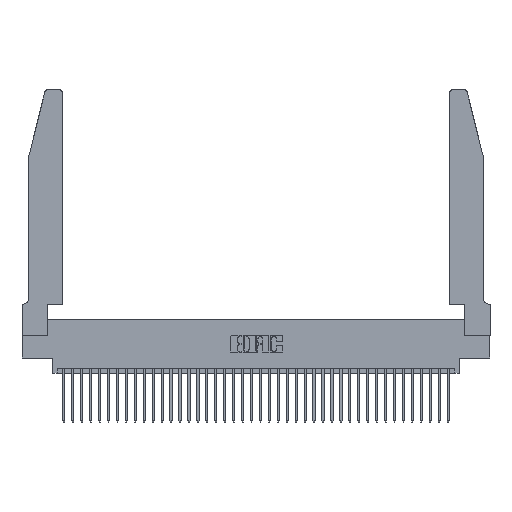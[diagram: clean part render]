
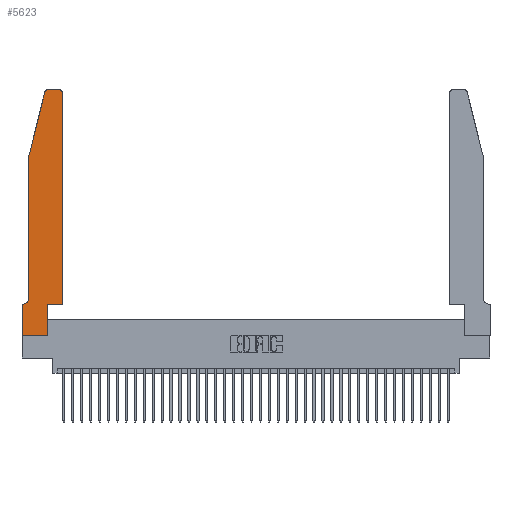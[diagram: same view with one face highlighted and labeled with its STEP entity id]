
A CAD part, top view. The second image highlights one B-rep face of the part: STEP entity #5623.
In plain terms, the highlighted planar face has unit normal (0, 0, 1).
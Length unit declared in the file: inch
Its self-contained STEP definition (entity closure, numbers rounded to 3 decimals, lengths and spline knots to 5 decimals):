
#653 = VERTEX_POINT ( 'NONE', #10343 ) ;
#885 = EDGE_CURVE ( 'NONE', #4570, #23562, #22742, .T. ) ;
#915 = ORIENTED_EDGE ( 'NONE', *, *, #18778, .T. ) ;
#2082 = VERTEX_POINT ( 'NONE', #32056 ) ;
#2391 = ORIENTED_EDGE ( 'NONE', *, *, #9731, .T. ) ;
#2848 = LINE ( 'NONE', #17155, #34085 ) ;
#3186 = AXIS2_PLACEMENT_3D ( 'NONE', #27260, #9106, #30260 ) ;
#3385 = EDGE_CURVE ( 'NONE', #26165, #33886, #33449, .T. ) ;
#4570 = VERTEX_POINT ( 'NONE', #22131 ) ;
#4640 = CARTESIAN_POINT ( 'NONE',  ( 0.4505, 0.35, 0.37 ) ) ;
#5017 = ORIENTED_EDGE ( 'NONE', *, *, #28313, .T. ) ;
#5269 = ORIENTED_EDGE ( 'NONE', *, *, #17800, .T. ) ;
#5487 = VECTOR ( 'NONE', #11917, 39.37008 ) ;
#5623 = ADVANCED_FACE ( 'NONE', ( #19562 ), #10812, .T. ) ;
#6093 = DIRECTION ( 'NONE',  ( 0., 1., 0. ) ) ;
#6188 = CIRCLE ( 'NONE', #3186, 0.03 ) ;
#6867 = DIRECTION ( 'NONE',  ( 0., -1., 0. ) ) ;
#7046 = ORIENTED_EDGE ( 'NONE', *, *, #26866, .T. ) ;
#7312 = VERTEX_POINT ( 'NONE', #31315 ) ;
#7690 = CARTESIAN_POINT ( 'NONE',  ( 0., 0., 0.37 ) ) ;
#7928 = ORIENTED_EDGE ( 'NONE', *, *, #30636, .T. ) ;
#8255 = AXIS2_PLACEMENT_3D ( 'NONE', #25917, #16947, #37991 ) ;
#9106 = DIRECTION ( 'NONE',  ( 0., 0., 1. ) ) ;
#9731 = EDGE_CURVE ( 'NONE', #33886, #15932, #36236, .T. ) ;
#10343 = CARTESIAN_POINT ( 'NONE',  ( 0.4505, 2.72, 0.37 ) ) ;
#10667 = DIRECTION ( 'NONE',  ( -0.239, -0.971, 0. ) ) ;
#10812 = PLANE ( 'NONE',  #8255 ) ;
#11277 = LINE ( 'NONE', #30303, #26446 ) ;
#11446 = EDGE_LOOP ( 'NONE', ( #12245, #7928, #19977, #2391, #16658, #7046, #21748, #12321, #37662, #5017, #915, #5269 ) ) ;
#11917 = DIRECTION ( 'NONE',  ( 1., 0., 0. ) ) ;
#12142 = VECTOR ( 'NONE', #6867, 39.37008 ) ;
#12245 = ORIENTED_EDGE ( 'NONE', *, *, #39118, .T. ) ;
#12321 = ORIENTED_EDGE ( 'NONE', *, *, #14594, .T. ) ;
#12380 = DIRECTION ( 'NONE',  ( 1., 0., 0. ) ) ;
#12825 = LINE ( 'NONE', #32810, #20917 ) ;
#13267 = VERTEX_POINT ( 'NONE', #18926 ) ;
#14496 = DIRECTION ( 'NONE',  ( 0., -1., 0. ) ) ;
#14589 = CIRCLE ( 'NONE', #16469, 0.03 ) ;
#14594 = EDGE_CURVE ( 'NONE', #23562, #2082, #30591, .T. ) ;
#14707 = VECTOR ( 'NONE', #14496, 39.37008 ) ;
#14733 = DIRECTION ( 'NONE',  ( -1., 0., 0. ) ) ;
#14947 = CIRCLE ( 'NONE', #24427, 0.07 ) ;
#14969 = CARTESIAN_POINT ( 'NONE',  ( 0.284, 2.72, 0.37 ) ) ;
#15932 = VERTEX_POINT ( 'NONE', #34512 ) ;
#16184 = DIRECTION ( 'NONE',  ( 0., 0., -1. ) ) ;
#16469 = AXIS2_PLACEMENT_3D ( 'NONE', #14969, #36056, #18043 ) ;
#16658 = ORIENTED_EDGE ( 'NONE', *, *, #36679, .T. ) ;
#16800 = CARTESIAN_POINT ( 'NONE',  ( 0.0755, 2., 0.37 ) ) ;
#16870 = DIRECTION ( 'NONE',  ( -1., 0., 0. ) ) ;
#16947 = DIRECTION ( 'NONE',  ( 0., 0., 1. ) ) ;
#17155 = CARTESIAN_POINT ( 'NONE',  ( 0.4505, 0.35, 0.37 ) ) ;
#17800 = EDGE_CURVE ( 'NONE', #653, #19831, #6188, .T. ) ;
#18043 = DIRECTION ( 'NONE',  ( 1., 0., 0. ) ) ;
#18778 = EDGE_CURVE ( 'NONE', #21673, #653, #2848, .T. ) ;
#18821 = CARTESIAN_POINT ( 'NONE',  ( 0.4205, 2.75, 0.37 ) ) ;
#18926 = CARTESIAN_POINT ( 'NONE',  ( 0.0055, 0.35, 0.37 ) ) ;
#19086 = CARTESIAN_POINT ( 'NONE',  ( 0.0755, 2., 0.37 ) ) ;
#19554 = CARTESIAN_POINT ( 'NONE',  ( 0.25487, 2.72718, 0.37 ) ) ;
#19562 = FACE_OUTER_BOUND ( 'NONE', #11446, .T. ) ;
#19689 = CARTESIAN_POINT ( 'NONE',  ( 0.0755, 2., 0.37 ) ) ;
#19831 = VERTEX_POINT ( 'NONE', #18821 ) ;
#19977 = ORIENTED_EDGE ( 'NONE', *, *, #3385, .T. ) ;
#20185 = DIRECTION ( 'NONE',  ( 0., 1., 0. ) ) ;
#20917 = VECTOR ( 'NONE', #14733, 39.37008 ) ;
#20954 = CARTESIAN_POINT ( 'NONE',  ( 0., 0., 0.37 ) ) ;
#21673 = VERTEX_POINT ( 'NONE', #4640 ) ;
#21748 = ORIENTED_EDGE ( 'NONE', *, *, #885, .T. ) ;
#22131 = CARTESIAN_POINT ( 'NONE',  ( 0., 0.35, 0.37 ) ) ;
#22264 = VECTOR ( 'NONE', #12380, 39.37008 ) ;
#22742 = LINE ( 'NONE', #23484, #14707 ) ;
#23233 = LINE ( 'NONE', #30482, #22264 ) ;
#23484 = CARTESIAN_POINT ( 'NONE',  ( 0., 0., 0.37 ) ) ;
#23562 = VERTEX_POINT ( 'NONE', #7690 ) ;
#23804 = EDGE_CURVE ( 'NONE', #2082, #7312, #11277, .T. ) ;
#24427 = AXIS2_PLACEMENT_3D ( 'NONE', #34244, #16184, #37247 ) ;
#25444 = VECTOR ( 'NONE', #10667, 39.37008 ) ;
#25917 = CARTESIAN_POINT ( 'NONE',  ( 0., 0.35, 0.37 ) ) ;
#26165 = VERTEX_POINT ( 'NONE', #19554 ) ;
#26446 = VECTOR ( 'NONE', #6093, 39.37008 ) ;
#26866 = EDGE_CURVE ( 'NONE', #13267, #4570, #27136, .T. ) ;
#27136 = LINE ( 'NONE', #34922, #35113 ) ;
#27260 = CARTESIAN_POINT ( 'NONE',  ( 0.4205, 2.72, 0.37 ) ) ;
#28313 = EDGE_CURVE ( 'NONE', #7312, #21673, #23233, .T. ) ;
#29083 = VERTEX_POINT ( 'NONE', #34054 ) ;
#30260 = DIRECTION ( 'NONE',  ( 1., 0., 0. ) ) ;
#30303 = CARTESIAN_POINT ( 'NONE',  ( 0.2865, 0.35, 0.37 ) ) ;
#30482 = CARTESIAN_POINT ( 'NONE',  ( 0.4505, 0.35, 0.37 ) ) ;
#30591 = LINE ( 'NONE', #20954, #5487 ) ;
#30636 = EDGE_CURVE ( 'NONE', #29083, #26165, #14589, .T. ) ;
#31315 = CARTESIAN_POINT ( 'NONE',  ( 0.2865, 0.35, 0.37 ) ) ;
#32056 = CARTESIAN_POINT ( 'NONE',  ( 0.2865, 0., 0.37 ) ) ;
#32810 = CARTESIAN_POINT ( 'NONE',  ( 0.2605, 2.75, 0.37 ) ) ;
#33449 = LINE ( 'NONE', #16800, #25444 ) ;
#33886 = VERTEX_POINT ( 'NONE', #19689 ) ;
#34054 = CARTESIAN_POINT ( 'NONE',  ( 0.284, 2.75, 0.37 ) ) ;
#34085 = VECTOR ( 'NONE', #20185, 39.37008 ) ;
#34244 = CARTESIAN_POINT ( 'NONE',  ( 0.0055, 0.42, 0.37 ) ) ;
#34512 = CARTESIAN_POINT ( 'NONE',  ( 0.0755, 0.42, 0.37 ) ) ;
#34922 = CARTESIAN_POINT ( 'NONE',  ( 0.0755, 0.35, 0.37 ) ) ;
#35113 = VECTOR ( 'NONE', #16870, 39.37008 ) ;
#36056 = DIRECTION ( 'NONE',  ( 0., 0., 1. ) ) ;
#36236 = LINE ( 'NONE', #19086, #12142 ) ;
#36679 = EDGE_CURVE ( 'NONE', #15932, #13267, #14947, .T. ) ;
#37247 = DIRECTION ( 'NONE',  ( -1., 0., 0. ) ) ;
#37662 = ORIENTED_EDGE ( 'NONE', *, *, #23804, .T. ) ;
#37991 = DIRECTION ( 'NONE',  ( 1., 0., 0. ) ) ;
#39118 = EDGE_CURVE ( 'NONE', #19831, #29083, #12825, .T. ) ;
